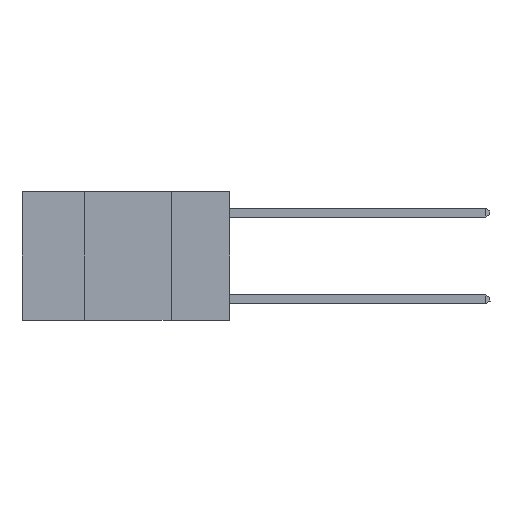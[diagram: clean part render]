
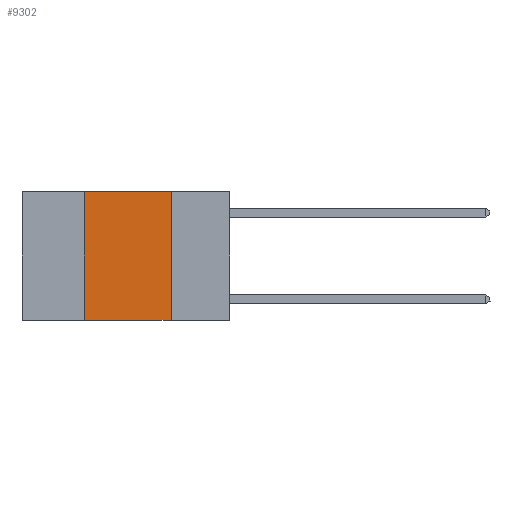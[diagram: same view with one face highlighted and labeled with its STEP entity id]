
A CAD part, left-side view. The second image highlights one B-rep face of the part: STEP entity #9302.
In plain terms, the highlighted planar face has unit normal (-1, 0, 0).
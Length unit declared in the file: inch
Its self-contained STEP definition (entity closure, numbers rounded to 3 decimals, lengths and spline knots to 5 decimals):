
#1090 = VECTOR ( 'NONE', #10949, 39.37008 ) ;
#1382 = ORIENTED_EDGE ( 'NONE', *, *, #13642, .F. ) ;
#2788 = DIRECTION ( 'NONE',  ( 0., -1., 0. ) ) ;
#3139 = CARTESIAN_POINT ( 'NONE',  ( 0., 0.17, -0.37 ) ) ;
#3189 = CARTESIAN_POINT ( 'NONE',  ( 0., 0.42, 0. ) ) ;
#4209 = EDGE_LOOP ( 'NONE', ( #10485, #13601, #1382, #15130 ) ) ;
#4883 = VECTOR ( 'NONE', #2788, 39.37008 ) ;
#5407 = LINE ( 'NONE', #12735, #4883 ) ;
#5576 = VERTEX_POINT ( 'NONE', #3189 ) ;
#5635 = CARTESIAN_POINT ( 'NONE',  ( 0., 0.6, 0. ) ) ;
#6167 = VERTEX_POINT ( 'NONE', #3139 ) ;
#7407 = EDGE_CURVE ( 'NONE', #8319, #6167, #5407, .T. ) ;
#7616 = VECTOR ( 'NONE', #20558, 39.37008 ) ;
#7805 = PLANE ( 'NONE',  #18957 ) ;
#8319 = VERTEX_POINT ( 'NONE', #11767 ) ;
#9302 = ADVANCED_FACE ( 'NONE', ( #12875 ), #7805, .F. ) ;
#9464 = CARTESIAN_POINT ( 'NONE',  ( 0., 0.6, 0. ) ) ;
#9667 = CARTESIAN_POINT ( 'NONE',  ( 0., 0.17, 0. ) ) ;
#10485 = ORIENTED_EDGE ( 'NONE', *, *, #14835, .F. ) ;
#10949 = DIRECTION ( 'NONE',  ( 0., 0., -1. ) ) ;
#11102 = DIRECTION ( 'NONE',  ( 0., 0., -1. ) ) ;
#11211 = DIRECTION ( 'NONE',  ( 0., 0., 1. ) ) ;
#11386 = VERTEX_POINT ( 'NONE', #9667 ) ;
#11767 = CARTESIAN_POINT ( 'NONE',  ( 0., 0.42, -0.37 ) ) ;
#12735 = CARTESIAN_POINT ( 'NONE',  ( 0., 0.6, -0.37 ) ) ;
#12875 = FACE_OUTER_BOUND ( 'NONE', #4209, .T. ) ;
#12959 = CARTESIAN_POINT ( 'NONE',  ( 0., 0.42, 0. ) ) ;
#13367 = LINE ( 'NONE', #12959, #17745 ) ;
#13601 = ORIENTED_EDGE ( 'NONE', *, *, #15773, .F. ) ;
#13642 = EDGE_CURVE ( 'NONE', #8319, #5576, #13367, .T. ) ;
#14835 = EDGE_CURVE ( 'NONE', #11386, #6167, #18209, .T. ) ;
#15130 = ORIENTED_EDGE ( 'NONE', *, *, #7407, .T. ) ;
#15773 = EDGE_CURVE ( 'NONE', #5576, #11386, #17424, .T. ) ;
#17424 = LINE ( 'NONE', #5635, #7616 ) ;
#17745 = VECTOR ( 'NONE', #11211, 39.37008 ) ;
#18209 = LINE ( 'NONE', #19194, #1090 ) ;
#18957 = AXIS2_PLACEMENT_3D ( 'NONE', #9464, #21053, #11102 ) ;
#19194 = CARTESIAN_POINT ( 'NONE',  ( 0., 0.17, 0. ) ) ;
#20558 = DIRECTION ( 'NONE',  ( 0., -1., 0. ) ) ;
#21053 = DIRECTION ( 'NONE',  ( 1., 0., 0. ) ) ;
